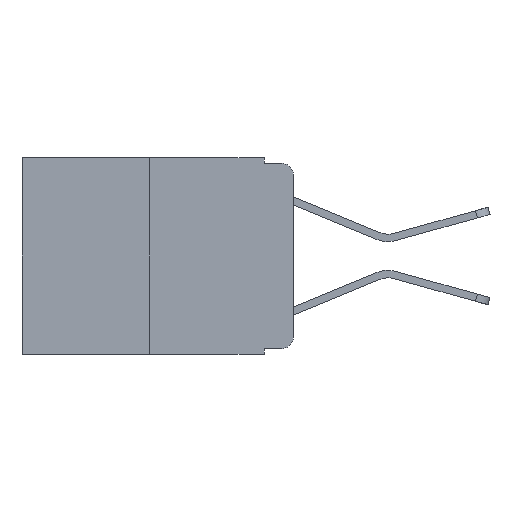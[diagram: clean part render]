
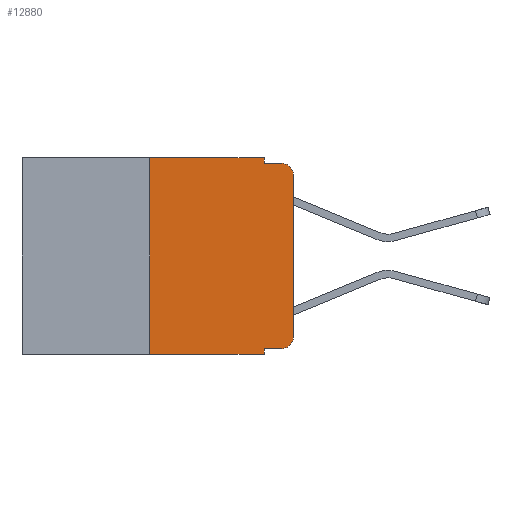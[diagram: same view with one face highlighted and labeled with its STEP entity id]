
A CAD part, left-side view. The second image highlights one B-rep face of the part: STEP entity #12880.
In plain terms, the highlighted planar face has unit normal (-1, 0, 0).
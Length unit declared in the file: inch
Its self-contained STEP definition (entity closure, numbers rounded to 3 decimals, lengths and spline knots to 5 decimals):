
#58 = VERTEX_POINT ( 'NONE', #21187 ) ;
#162 = DIRECTION ( 'NONE',  ( 0., 0., -1. ) ) ;
#466 = PLANE ( 'NONE',  #22457 ) ;
#1666 = CARTESIAN_POINT ( 'NONE',  ( 0., 0.473, 0. ) ) ;
#1990 = EDGE_CURVE ( 'NONE', #16229, #11154, #6576, .T. ) ;
#2346 = LINE ( 'NONE', #1666, #3537 ) ;
#2464 = EDGE_CURVE ( 'NONE', #11154, #19141, #21585, .T. ) ;
#2891 = CARTESIAN_POINT ( 'NONE',  ( 0., 0.051, -0.343 ) ) ;
#3163 = LINE ( 'NONE', #22285, #21446 ) ;
#3176 = VECTOR ( 'NONE', #18047, 39.37008 ) ;
#3537 = VECTOR ( 'NONE', #14637, 39.37008 ) ;
#3561 = ORIENTED_EDGE ( 'NONE', *, *, #14102, .F. ) ;
#3899 = CARTESIAN_POINT ( 'NONE',  ( 0., 0.02, -0.333 ) ) ;
#4891 = CARTESIAN_POINT ( 'NONE',  ( 0., 0.02, -0.01 ) ) ;
#5049 = LINE ( 'NONE', #5940, #23223 ) ;
#5123 = EDGE_CURVE ( 'NONE', #18554, #8270, #5049, .T. ) ;
#5452 = CARTESIAN_POINT ( 'NONE',  ( 0., 0.25, 0. ) ) ;
#5533 = VECTOR ( 'NONE', #9245, 39.37008 ) ;
#5847 = VERTEX_POINT ( 'NONE', #11406 ) ;
#5940 = CARTESIAN_POINT ( 'NONE',  ( 0., 0.473, -0.343 ) ) ;
#6182 = DIRECTION ( 'NONE',  ( 1., 0., 0. ) ) ;
#6402 = CARTESIAN_POINT ( 'NONE',  ( 0., 0.25, -0.343 ) ) ;
#6504 = CARTESIAN_POINT ( 'NONE',  ( 0., 0.051, -0.01 ) ) ;
#6576 = LINE ( 'NONE', #22859, #21058 ) ;
#7150 = CARTESIAN_POINT ( 'NONE',  ( 0., 0.051, 0. ) ) ;
#7485 = CARTESIAN_POINT ( 'NONE',  ( 0., 0.02, -0.03 ) ) ;
#7783 = VERTEX_POINT ( 'NONE', #20038 ) ;
#7849 = DIRECTION ( 'NONE',  ( -1., 0., 0. ) ) ;
#7901 = DIRECTION ( 'NONE',  ( 0., -1., 0. ) ) ;
#7991 = EDGE_CURVE ( 'NONE', #19141, #58, #3163, .T. ) ;
#8270 = VERTEX_POINT ( 'NONE', #2891 ) ;
#9245 = DIRECTION ( 'NONE',  ( 0., 0., 1. ) ) ;
#9354 = DIRECTION ( 'NONE',  ( 0., 0., -1. ) ) ;
#9554 = CARTESIAN_POINT ( 'NONE',  ( 0., 0.051, 0. ) ) ;
#9721 = ORIENTED_EDGE ( 'NONE', *, *, #10448, .T. ) ;
#9741 = VERTEX_POINT ( 'NONE', #21848 ) ;
#9970 = EDGE_LOOP ( 'NONE', ( #15833, #9721, #17631, #3561, #17477, #14484, #16610, #14719, #14906, #19064 ) ) ;
#10448 = EDGE_CURVE ( 'NONE', #58, #10860, #19537, .T. ) ;
#10860 = VERTEX_POINT ( 'NONE', #4891 ) ;
#11154 = VERTEX_POINT ( 'NONE', #3899 ) ;
#11279 = FACE_OUTER_BOUND ( 'NONE', #9970, .T. ) ;
#11406 = CARTESIAN_POINT ( 'NONE',  ( 0., 0.051, 0. ) ) ;
#11702 = EDGE_CURVE ( 'NONE', #7783, #10860, #13307, .T. ) ;
#12142 = DIRECTION ( 'NONE',  ( 0., 0., -1. ) ) ;
#12846 = AXIS2_PLACEMENT_3D ( 'NONE', #7485, #20173, #9354 ) ;
#12880 = ADVANCED_FACE ( 'NONE', ( #11279 ), #466, .F. ) ;
#13307 = LINE ( 'NONE', #6504, #18079 ) ;
#13439 = CARTESIAN_POINT ( 'NONE',  ( 0., 0.473, 0. ) ) ;
#14102 = EDGE_CURVE ( 'NONE', #5847, #7783, #23500, .T. ) ;
#14484 = ORIENTED_EDGE ( 'NONE', *, *, #18891, .F. ) ;
#14637 = DIRECTION ( 'NONE',  ( 0., -1., 0. ) ) ;
#14719 = ORIENTED_EDGE ( 'NONE', *, *, #20121, .F. ) ;
#14906 = ORIENTED_EDGE ( 'NONE', *, *, #1990, .T. ) ;
#15833 = ORIENTED_EDGE ( 'NONE', *, *, #7991, .T. ) ;
#15898 = LINE ( 'NONE', #5452, #5533 ) ;
#16229 = VERTEX_POINT ( 'NONE', #21355 ) ;
#16610 = ORIENTED_EDGE ( 'NONE', *, *, #5123, .T. ) ;
#17249 = AXIS2_PLACEMENT_3D ( 'NONE', #19257, #7849, #12142 ) ;
#17432 = DIRECTION ( 'NONE',  ( 0., -1., 0. ) ) ;
#17477 = ORIENTED_EDGE ( 'NONE', *, *, #22038, .F. ) ;
#17631 = ORIENTED_EDGE ( 'NONE', *, *, #11702, .F. ) ;
#18047 = DIRECTION ( 'NONE',  ( 0., 0., -1. ) ) ;
#18079 = VECTOR ( 'NONE', #17432, 39.37008 ) ;
#18382 = LINE ( 'NONE', #7150, #3176 ) ;
#18554 = VERTEX_POINT ( 'NONE', #6402 ) ;
#18787 = VECTOR ( 'NONE', #162, 39.37008 ) ;
#18891 = EDGE_CURVE ( 'NONE', #18554, #9741, #15898, .T. ) ;
#18906 = DIRECTION ( 'NONE',  ( 0., 0., -1. ) ) ;
#19064 = ORIENTED_EDGE ( 'NONE', *, *, #2464, .T. ) ;
#19141 = VERTEX_POINT ( 'NONE', #20684 ) ;
#19257 = CARTESIAN_POINT ( 'NONE',  ( 0., 0.02, -0.313 ) ) ;
#19537 = CIRCLE ( 'NONE', #12846, 0.02 ) ;
#20038 = CARTESIAN_POINT ( 'NONE',  ( 0., 0.051, -0.01 ) ) ;
#20121 = EDGE_CURVE ( 'NONE', #16229, #8270, #18382, .T. ) ;
#20173 = DIRECTION ( 'NONE',  ( -1., 0., 0. ) ) ;
#20582 = DIRECTION ( 'NONE',  ( 0., 0., 1. ) ) ;
#20684 = CARTESIAN_POINT ( 'NONE',  ( 0., 0., -0.313 ) ) ;
#21058 = VECTOR ( 'NONE', #22791, 39.37008 ) ;
#21187 = CARTESIAN_POINT ( 'NONE',  ( 0., 0., -0.03 ) ) ;
#21355 = CARTESIAN_POINT ( 'NONE',  ( 0., 0.051, -0.333 ) ) ;
#21446 = VECTOR ( 'NONE', #20582, 39.37008 ) ;
#21585 = CIRCLE ( 'NONE', #17249, 0.02 ) ;
#21848 = CARTESIAN_POINT ( 'NONE',  ( 0., 0.25, 0. ) ) ;
#22038 = EDGE_CURVE ( 'NONE', #9741, #5847, #2346, .T. ) ;
#22285 = CARTESIAN_POINT ( 'NONE',  ( 0., 0., 0. ) ) ;
#22457 = AXIS2_PLACEMENT_3D ( 'NONE', #13439, #6182, #18906 ) ;
#22791 = DIRECTION ( 'NONE',  ( 0., -1., 0. ) ) ;
#22859 = CARTESIAN_POINT ( 'NONE',  ( 0., 0.051, -0.333 ) ) ;
#23223 = VECTOR ( 'NONE', #7901, 39.37008 ) ;
#23500 = LINE ( 'NONE', #9554, #18787 ) ;
